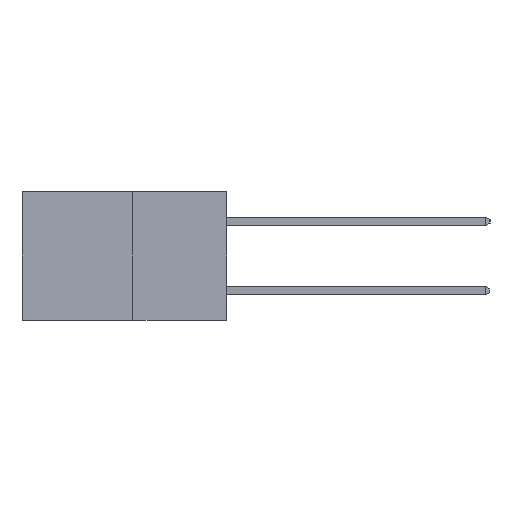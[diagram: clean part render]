
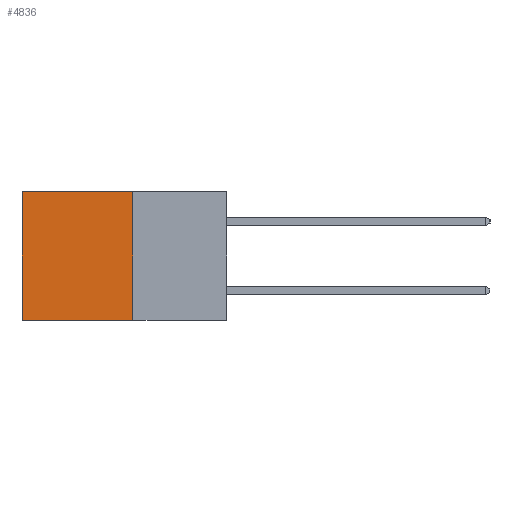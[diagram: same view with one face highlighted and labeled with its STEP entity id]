
A CAD part, left-side view. The second image highlights one B-rep face of the part: STEP entity #4836.
In plain terms, the highlighted planar face has unit normal (-1, 0, 0).
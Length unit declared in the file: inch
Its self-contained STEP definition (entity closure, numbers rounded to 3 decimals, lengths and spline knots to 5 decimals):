
#1 = CARTESIAN_POINT ( 'NONE',  ( 0.277, 0.27, -0.37 ) ) ;
#108 = DIRECTION ( 'NONE',  ( 0., 0., -1. ) ) ;
#416 = CARTESIAN_POINT ( 'NONE',  ( 0.277, 0.59, -0.37 ) ) ;
#517 = VECTOR ( 'NONE', #108, 39.37008 ) ;
#828 = ORIENTED_EDGE ( 'NONE', *, *, #1580, .T. ) ;
#1161 = CARTESIAN_POINT ( 'NONE',  ( 0.277, 0.27, 0. ) ) ;
#1281 = LINE ( 'NONE', #1161, #8380 ) ;
#1580 = EDGE_CURVE ( 'NONE', #6545, #1715, #4514, .T. ) ;
#1715 = VERTEX_POINT ( 'NONE', #3247 ) ;
#1825 = EDGE_CURVE ( 'NONE', #5251, #6545, #1281, .T. ) ;
#2087 = DIRECTION ( 'NONE',  ( 0., 1., 0. ) ) ;
#2248 = VECTOR ( 'NONE', #2087, 39.37008 ) ;
#3247 = CARTESIAN_POINT ( 'NONE',  ( 0.277, 0.59, -0.37 ) ) ;
#3455 = CARTESIAN_POINT ( 'NONE',  ( 0.277, 0.27, -0.37 ) ) ;
#3746 = AXIS2_PLACEMENT_3D ( 'NONE', #5275, #4913, #8240 ) ;
#3901 = ORIENTED_EDGE ( 'NONE', *, *, #6502, .F. ) ;
#4281 = EDGE_LOOP ( 'NONE', ( #828, #6269, #3901, #7233 ) ) ;
#4514 = LINE ( 'NONE', #416, #517 ) ;
#4751 = EDGE_CURVE ( 'NONE', #5476, #1715, #6454, .T. ) ;
#4836 = ADVANCED_FACE ( 'NONE', ( #7902 ), #7484, .F. ) ;
#4913 = DIRECTION ( 'NONE',  ( 1., 0., 0. ) ) ;
#5251 = VERTEX_POINT ( 'NONE', #7029 ) ;
#5275 = CARTESIAN_POINT ( 'NONE',  ( 0.277, 0.27, -0.37 ) ) ;
#5372 = DIRECTION ( 'NONE',  ( 0., 1., 0. ) ) ;
#5476 = VERTEX_POINT ( 'NONE', #7942 ) ;
#5919 = CARTESIAN_POINT ( 'NONE',  ( 0.277, 0.59, 0. ) ) ;
#6269 = ORIENTED_EDGE ( 'NONE', *, *, #4751, .F. ) ;
#6364 = LINE ( 'NONE', #1, #6558 ) ;
#6454 = LINE ( 'NONE', #3455, #2248 ) ;
#6502 = EDGE_CURVE ( 'NONE', #5251, #5476, #6364, .T. ) ;
#6545 = VERTEX_POINT ( 'NONE', #5919 ) ;
#6558 = VECTOR ( 'NONE', #7184, 39.37008 ) ;
#7029 = CARTESIAN_POINT ( 'NONE',  ( 0.277, 0.27, 0. ) ) ;
#7184 = DIRECTION ( 'NONE',  ( 0., 0., -1. ) ) ;
#7233 = ORIENTED_EDGE ( 'NONE', *, *, #1825, .T. ) ;
#7484 = PLANE ( 'NONE',  #3746 ) ;
#7902 = FACE_OUTER_BOUND ( 'NONE', #4281, .T. ) ;
#7942 = CARTESIAN_POINT ( 'NONE',  ( 0.277, 0.27, -0.37 ) ) ;
#8240 = DIRECTION ( 'NONE',  ( 0., 0., -1. ) ) ;
#8380 = VECTOR ( 'NONE', #5372, 39.37008 ) ;
